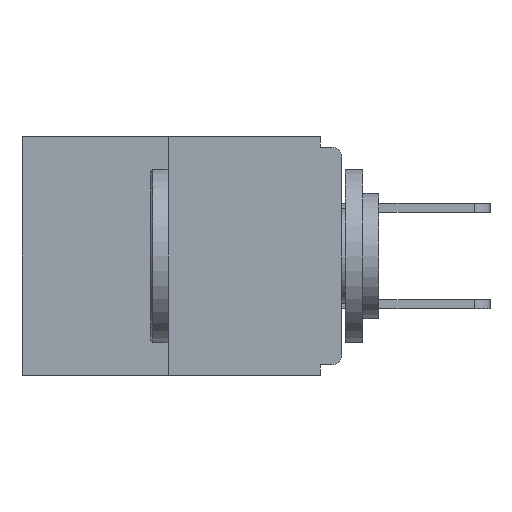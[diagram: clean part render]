
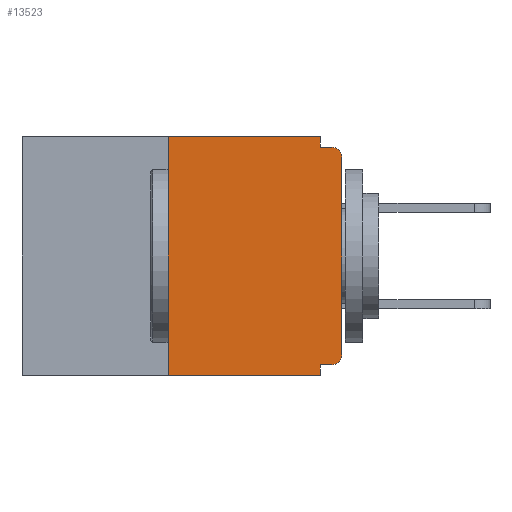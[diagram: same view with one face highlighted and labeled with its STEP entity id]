
A CAD part, left-side view. The second image highlights one B-rep face of the part: STEP entity #13523.
In plain terms, the highlighted planar face has unit normal (-1, 0, 0).
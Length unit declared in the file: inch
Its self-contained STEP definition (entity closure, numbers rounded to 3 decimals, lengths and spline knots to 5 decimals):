
#219 = CARTESIAN_POINT ( 'NONE',  ( 0., 0.031, -0.343 ) ) ;
#883 = ORIENTED_EDGE ( 'NONE', *, *, #9074, .F. ) ;
#1082 = FACE_OUTER_BOUND ( 'NONE', #7351, .T. ) ;
#1247 = VECTOR ( 'NONE', #12622, 39.37008 ) ;
#1271 = LINE ( 'NONE', #17633, #16336 ) ;
#1470 = CARTESIAN_POINT ( 'NONE',  ( 0., 0.031, -0.343 ) ) ;
#1538 = LINE ( 'NONE', #18735, #19827 ) ;
#1693 = ORIENTED_EDGE ( 'NONE', *, *, #5412, .F. ) ;
#1724 = CARTESIAN_POINT ( 'NONE',  ( 0., 0.46, 0. ) ) ;
#1778 = CARTESIAN_POINT ( 'NONE',  ( 0., 0.031, 0. ) ) ;
#1785 = LINE ( 'NONE', #6643, #10121 ) ;
#1801 = LINE ( 'NONE', #16505, #21253 ) ;
#2122 = CIRCLE ( 'NONE', #19252, 0.015 ) ;
#2163 = CARTESIAN_POINT ( 'NONE',  ( 0., 0.015, -0.313 ) ) ;
#2223 = AXIS2_PLACEMENT_3D ( 'NONE', #17057, #18837, #11242 ) ;
#2303 = CARTESIAN_POINT ( 'NONE',  ( 0., 0.015, -0.328 ) ) ;
#2772 = VECTOR ( 'NONE', #16827, 39.37008 ) ;
#2846 = VERTEX_POINT ( 'NONE', #7771 ) ;
#4591 = EDGE_CURVE ( 'NONE', #11056, #17723, #15518, .T. ) ;
#4807 = VECTOR ( 'NONE', #20860, 39.37008 ) ;
#4994 = VERTEX_POINT ( 'NONE', #11264 ) ;
#5299 = CARTESIAN_POINT ( 'NONE',  ( 0., 0., -0.328 ) ) ;
#5412 = EDGE_CURVE ( 'NONE', #17723, #17455, #8400, .T. ) ;
#5508 = VERTEX_POINT ( 'NONE', #5959 ) ;
#5652 = EDGE_CURVE ( 'NONE', #22249, #4994, #1271, .T. ) ;
#5959 = CARTESIAN_POINT ( 'NONE',  ( 0., 0.015, -0.015 ) ) ;
#6457 = EDGE_CURVE ( 'NONE', #17455, #16507, #1538, .T. ) ;
#6643 = CARTESIAN_POINT ( 'NONE',  ( 0., 0., -0.015 ) ) ;
#7351 = EDGE_LOOP ( 'NONE', ( #1693, #15058, #8530, #883, #7636, #15480, #8939, #19208, #22658, #22234 ) ) ;
#7636 = ORIENTED_EDGE ( 'NONE', *, *, #10176, .F. ) ;
#7771 = CARTESIAN_POINT ( 'NONE',  ( 0., 0.031, -0.328 ) ) ;
#7885 = EDGE_CURVE ( 'NONE', #16507, #5508, #1785, .T. ) ;
#7890 = PLANE ( 'NONE',  #23411 ) ;
#8201 = CARTESIAN_POINT ( 'NONE',  ( 0., 0., -0.313 ) ) ;
#8400 = LINE ( 'NONE', #1724, #2772 ) ;
#8530 = ORIENTED_EDGE ( 'NONE', *, *, #17795, .T. ) ;
#8939 = ORIENTED_EDGE ( 'NONE', *, *, #5652, .T. ) ;
#9005 = VECTOR ( 'NONE', #14918, 39.37008 ) ;
#9074 = EDGE_CURVE ( 'NONE', #2846, #17878, #9897, .T. ) ;
#9717 = VERTEX_POINT ( 'NONE', #2303 ) ;
#9897 = LINE ( 'NONE', #219, #4807 ) ;
#10121 = VECTOR ( 'NONE', #10705, 39.37008 ) ;
#10176 = EDGE_CURVE ( 'NONE', #9717, #2846, #13097, .T. ) ;
#10462 = EDGE_CURVE ( 'NONE', #9717, #22249, #2122, .T. ) ;
#10705 = DIRECTION ( 'NONE',  ( 0., -1., 0. ) ) ;
#10847 = DIRECTION ( 'NONE',  ( 0., -1., 0. ) ) ;
#11035 = EDGE_CURVE ( 'NONE', #4994, #5508, #11555, .T. ) ;
#11056 = VERTEX_POINT ( 'NONE', #14952 ) ;
#11242 = DIRECTION ( 'NONE',  ( 0., 0., -1. ) ) ;
#11264 = CARTESIAN_POINT ( 'NONE',  ( 0., 0., -0.03 ) ) ;
#11555 = CIRCLE ( 'NONE', #2223, 0.015 ) ;
#11867 = CARTESIAN_POINT ( 'NONE',  ( 0., 0.031, -0.015 ) ) ;
#12622 = DIRECTION ( 'NONE',  ( 0., 1., 0. ) ) ;
#13097 = LINE ( 'NONE', #5299, #1247 ) ;
#13523 = ADVANCED_FACE ( 'NONE', ( #1082 ), #7890, .F. ) ;
#14918 = DIRECTION ( 'NONE',  ( 0., 0., 1. ) ) ;
#14952 = CARTESIAN_POINT ( 'NONE',  ( 0., 0.25, -0.343 ) ) ;
#15058 = ORIENTED_EDGE ( 'NONE', *, *, #4591, .F. ) ;
#15257 = DIRECTION ( 'NONE',  ( 0., 0., -1. ) ) ;
#15390 = DIRECTION ( 'NONE',  ( -1., 0., 0. ) ) ;
#15417 = DIRECTION ( 'NONE',  ( 1., 0., 0. ) ) ;
#15480 = ORIENTED_EDGE ( 'NONE', *, *, #10462, .T. ) ;
#15518 = LINE ( 'NONE', #19956, #9005 ) ;
#16336 = VECTOR ( 'NONE', #23487, 39.37008 ) ;
#16505 = CARTESIAN_POINT ( 'NONE',  ( 0., 0.46, -0.343 ) ) ;
#16507 = VERTEX_POINT ( 'NONE', #11867 ) ;
#16827 = DIRECTION ( 'NONE',  ( 0., -1., 0. ) ) ;
#17057 = CARTESIAN_POINT ( 'NONE',  ( 0., 0.015, -0.03 ) ) ;
#17455 = VERTEX_POINT ( 'NONE', #1778 ) ;
#17633 = CARTESIAN_POINT ( 'NONE',  ( 0., 0., 0. ) ) ;
#17723 = VERTEX_POINT ( 'NONE', #19859 ) ;
#17795 = EDGE_CURVE ( 'NONE', #11056, #17878, #1801, .T. ) ;
#17878 = VERTEX_POINT ( 'NONE', #1470 ) ;
#18735 = CARTESIAN_POINT ( 'NONE',  ( 0., 0.031, 0. ) ) ;
#18837 = DIRECTION ( 'NONE',  ( -1., 0., 0. ) ) ;
#19040 = DIRECTION ( 'NONE',  ( 0., 0., -1. ) ) ;
#19208 = ORIENTED_EDGE ( 'NONE', *, *, #11035, .T. ) ;
#19252 = AXIS2_PLACEMENT_3D ( 'NONE', #2163, #15390, #19040 ) ;
#19827 = VECTOR ( 'NONE', #15257, 39.37008 ) ;
#19859 = CARTESIAN_POINT ( 'NONE',  ( 0., 0.25, 0. ) ) ;
#19956 = CARTESIAN_POINT ( 'NONE',  ( 0., 0.25, 0. ) ) ;
#20860 = DIRECTION ( 'NONE',  ( 0., 0., -1. ) ) ;
#21025 = CARTESIAN_POINT ( 'NONE',  ( 0., 0.46, 0. ) ) ;
#21253 = VECTOR ( 'NONE', #10847, 39.37008 ) ;
#22234 = ORIENTED_EDGE ( 'NONE', *, *, #6457, .F. ) ;
#22249 = VERTEX_POINT ( 'NONE', #8201 ) ;
#22658 = ORIENTED_EDGE ( 'NONE', *, *, #7885, .F. ) ;
#22718 = DIRECTION ( 'NONE',  ( 0., 0., -1. ) ) ;
#23411 = AXIS2_PLACEMENT_3D ( 'NONE', #21025, #15417, #22718 ) ;
#23487 = DIRECTION ( 'NONE',  ( 0., 0., 1. ) ) ;
